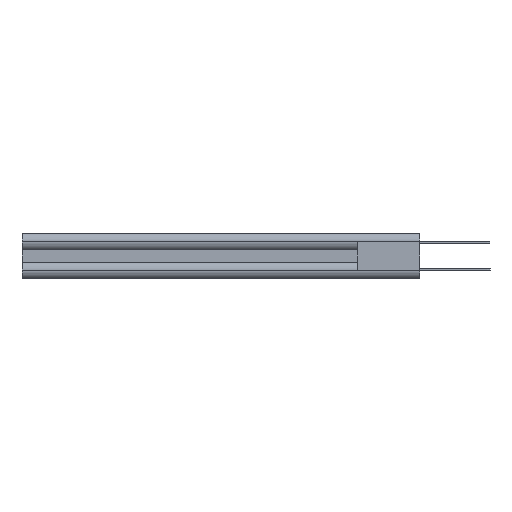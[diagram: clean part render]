
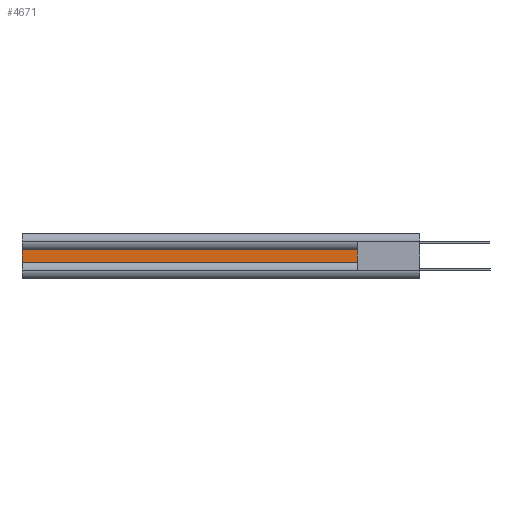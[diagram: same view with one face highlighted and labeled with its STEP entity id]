
A CAD part, left-side view. The second image highlights one B-rep face of the part: STEP entity #4671.
In plain terms, the highlighted planar face has unit normal (-1, 0, 0).
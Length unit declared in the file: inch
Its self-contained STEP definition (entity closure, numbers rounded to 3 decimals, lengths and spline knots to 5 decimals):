
#41 = LINE ( 'NONE', #4721, #8836 ) ;
#797 = FACE_OUTER_BOUND ( 'NONE', #12083, .T. ) ;
#1131 = CARTESIAN_POINT ( 'NONE',  ( 0.044, 0.37012, -0.0465 ) ) ;
#1196 = DIRECTION ( 'NONE',  ( 0., 0., -1. ) ) ;
#3536 = VERTEX_POINT ( 'NONE', #6675 ) ;
#3545 = DIRECTION ( 'NONE',  ( 0., 1., 0. ) ) ;
#3583 = CARTESIAN_POINT ( 'NONE',  ( 0.044, 3., -0.0465 ) ) ;
#4671 = ADVANCED_FACE ( 'NONE', ( #797 ), #18293, .F. ) ;
#4721 = CARTESIAN_POINT ( 'NONE',  ( 0.044, 3., -0.0465 ) ) ;
#4734 = EDGE_CURVE ( 'NONE', #18029, #3536, #8480, .T. ) ;
#4809 = DIRECTION ( 'NONE',  ( 0., 0., -1. ) ) ;
#4985 = ORIENTED_EDGE ( 'NONE', *, *, #4734, .F. ) ;
#6432 = DIRECTION ( 'NONE',  ( 1., 0., 0. ) ) ;
#6675 = CARTESIAN_POINT ( 'NONE',  ( 0.044, 0.473, -0.0465 ) ) ;
#8480 = LINE ( 'NONE', #13404, #13020 ) ;
#8791 = VECTOR ( 'NONE', #3545, 39.37008 ) ;
#8836 = VECTOR ( 'NONE', #1196, 39.37008 ) ;
#9113 = DIRECTION ( 'NONE',  ( 0., 1., 0. ) ) ;
#9714 = VERTEX_POINT ( 'NONE', #13570 ) ;
#10113 = LINE ( 'NONE', #17640, #18602 ) ;
#10261 = EDGE_CURVE ( 'NONE', #9714, #14712, #41, .T. ) ;
#11035 = EDGE_CURVE ( 'NONE', #18029, #9714, #14382, .T. ) ;
#11196 = EDGE_CURVE ( 'NONE', #3536, #14712, #10113, .T. ) ;
#11724 = AXIS2_PLACEMENT_3D ( 'NONE', #1131, #6432, #18357 ) ;
#12083 = EDGE_LOOP ( 'NONE', ( #21133, #16796, #14775, #4985 ) ) ;
#13020 = VECTOR ( 'NONE', #4809, 39.37008 ) ;
#13404 = CARTESIAN_POINT ( 'NONE',  ( 0.044, 0.473, -0.0465 ) ) ;
#13570 = CARTESIAN_POINT ( 'NONE',  ( 0.044, 3., 0.0465 ) ) ;
#14382 = LINE ( 'NONE', #17186, #8791 ) ;
#14712 = VERTEX_POINT ( 'NONE', #3583 ) ;
#14775 = ORIENTED_EDGE ( 'NONE', *, *, #11196, .F. ) ;
#16796 = ORIENTED_EDGE ( 'NONE', *, *, #10261, .T. ) ;
#17186 = CARTESIAN_POINT ( 'NONE',  ( 0.044, 0.37012, 0.0465 ) ) ;
#17640 = CARTESIAN_POINT ( 'NONE',  ( 0.044, 0.37012, -0.0465 ) ) ;
#18029 = VERTEX_POINT ( 'NONE', #21693 ) ;
#18293 = PLANE ( 'NONE',  #11724 ) ;
#18357 = DIRECTION ( 'NONE',  ( 0., 0., -1. ) ) ;
#18602 = VECTOR ( 'NONE', #9113, 39.37008 ) ;
#21133 = ORIENTED_EDGE ( 'NONE', *, *, #11035, .T. ) ;
#21693 = CARTESIAN_POINT ( 'NONE',  ( 0.044, 0.473, 0.0465 ) ) ;
